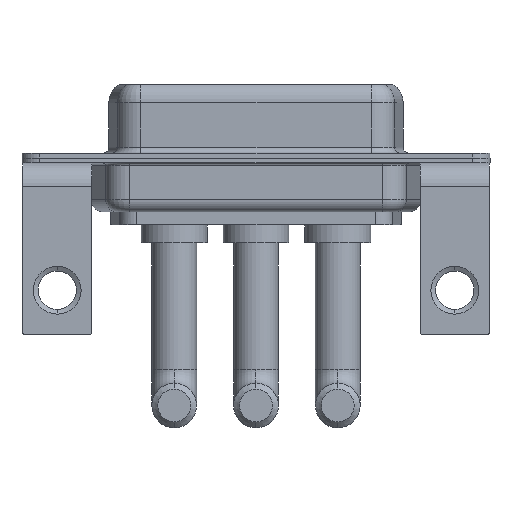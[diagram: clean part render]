
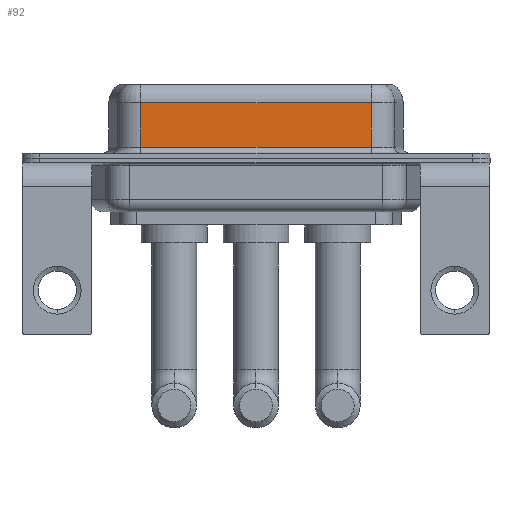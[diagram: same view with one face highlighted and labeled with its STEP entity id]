
A CAD part, front view. The second image highlights one B-rep face of the part: STEP entity #92.
In plain terms, the highlighted planar face has unit normal (0, -1, 0).
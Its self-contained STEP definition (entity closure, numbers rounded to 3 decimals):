
#92 = ADVANCED_FACE ( 'NONE', ( #3960 ), #5087, .F. ) ;
#185 = LINE ( 'NONE', #981, #11453 ) ;
#204 = LINE ( 'NONE', #9539, #6813 ) ;
#225 = EDGE_LOOP ( 'NONE', ( #2958, #2183, #9958, #8162 ) ) ;
#593 = VERTEX_POINT ( 'NONE', #8278 ) ;
#615 = CARTESIAN_POINT ( 'NONE',  ( 7.013, -3.95, 4.65 ) ) ;
#981 = CARTESIAN_POINT ( 'NONE',  ( 26.287, -3.95, 0.9 ) ) ;
#1063 = CARTESIAN_POINT ( 'NONE',  ( 26.287, -3.95, 6.4 ) ) ;
#1272 = DIRECTION ( 'NONE',  ( 0., 0., -1. ) ) ;
#1418 = EDGE_CURVE ( 'NONE', #5964, #593, #7793, .T. ) ;
#1520 = VECTOR ( 'NONE', #3525, 1000. ) ;
#1873 = CARTESIAN_POINT ( 'NONE',  ( 7.013, -3.95, 0.9 ) ) ;
#1962 = EDGE_CURVE ( 'NONE', #7398, #593, #185, .T. ) ;
#2183 = ORIENTED_EDGE ( 'NONE', *, *, #3351, .T. ) ;
#2784 = VERTEX_POINT ( 'NONE', #615 ) ;
#2958 = ORIENTED_EDGE ( 'NONE', *, *, #1418, .F. ) ;
#2989 = CARTESIAN_POINT ( 'NONE',  ( 26.287, -3.95, 6.4 ) ) ;
#3351 = EDGE_CURVE ( 'NONE', #5964, #2784, #5035, .T. ) ;
#3525 = DIRECTION ( 'NONE',  ( 0., 0., -1. ) ) ;
#3949 = DIRECTION ( 'NONE',  ( 1., 0., 0. ) ) ;
#3960 = FACE_OUTER_BOUND ( 'NONE', #225, .T. ) ;
#5035 = LINE ( 'NONE', #9095, #12080 ) ;
#5087 = PLANE ( 'NONE',  #6376 ) ;
#5178 = EDGE_CURVE ( 'NONE', #2784, #7398, #204, .T. ) ;
#5964 = VERTEX_POINT ( 'NONE', #6866 ) ;
#6376 = AXIS2_PLACEMENT_3D ( 'NONE', #1063, #8031, #12069 ) ;
#6813 = VECTOR ( 'NONE', #1272, 1000. ) ;
#6866 = CARTESIAN_POINT ( 'NONE',  ( 26.287, -3.95, 4.65 ) ) ;
#7398 = VERTEX_POINT ( 'NONE', #1873 ) ;
#7793 = LINE ( 'NONE', #2989, #1520 ) ;
#8031 = DIRECTION ( 'NONE',  ( 0., 1., 0. ) ) ;
#8114 = DIRECTION ( 'NONE',  ( -1., 0., 0. ) ) ;
#8162 = ORIENTED_EDGE ( 'NONE', *, *, #1962, .T. ) ;
#8278 = CARTESIAN_POINT ( 'NONE',  ( 26.287, -3.95, 0.9 ) ) ;
#9095 = CARTESIAN_POINT ( 'NONE',  ( 26.287, -3.95, 4.65 ) ) ;
#9539 = CARTESIAN_POINT ( 'NONE',  ( 7.013, -3.95, 6.4 ) ) ;
#9958 = ORIENTED_EDGE ( 'NONE', *, *, #5178, .T. ) ;
#11453 = VECTOR ( 'NONE', #3949, 1000. ) ;
#12069 = DIRECTION ( 'NONE',  ( 0., 0., 1. ) ) ;
#12080 = VECTOR ( 'NONE', #8114, 1000. ) ;
